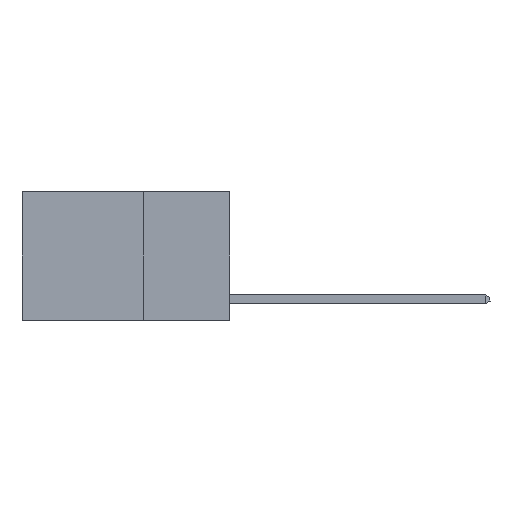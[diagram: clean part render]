
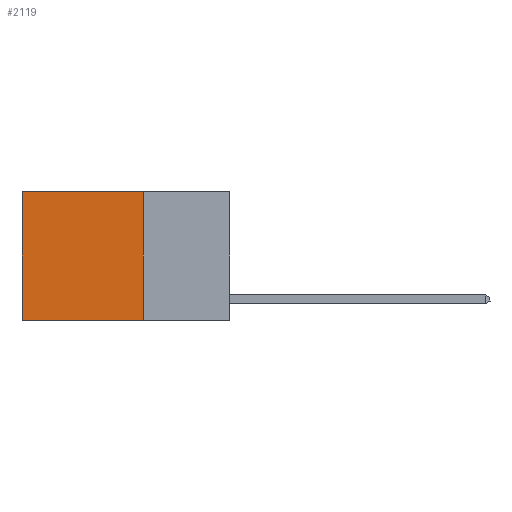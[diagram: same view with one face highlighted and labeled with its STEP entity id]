
A CAD part, left-side view. The second image highlights one B-rep face of the part: STEP entity #2119.
In plain terms, the highlighted planar face has unit normal (-1, 0, 0).
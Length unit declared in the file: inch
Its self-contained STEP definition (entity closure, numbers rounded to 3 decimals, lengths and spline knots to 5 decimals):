
#32 = EDGE_CURVE ( 'NONE', #3670, #4862, #2466, .T. ) ;
#75 = LINE ( 'NONE', #8526, #9297 ) ;
#230 = CARTESIAN_POINT ( 'NONE',  ( 0.2625, 0.25, 0. ) ) ;
#380 = ORIENTED_EDGE ( 'NONE', *, *, #10421, .T. ) ;
#608 = CARTESIAN_POINT ( 'NONE',  ( 0.2625, 0.25, 0. ) ) ;
#822 = CARTESIAN_POINT ( 'NONE',  ( 0.2625, 0.6, -0.37 ) ) ;
#2119 = ADVANCED_FACE ( 'NONE', ( #2214 ), #14959, .F. ) ;
#2214 = FACE_OUTER_BOUND ( 'NONE', #12227, .T. ) ;
#2344 = VERTEX_POINT ( 'NONE', #12533 ) ;
#2466 = LINE ( 'NONE', #230, #11233 ) ;
#3179 = ORIENTED_EDGE ( 'NONE', *, *, #32, .F. ) ;
#3670 = VERTEX_POINT ( 'NONE', #608 ) ;
#4862 = VERTEX_POINT ( 'NONE', #7454 ) ;
#5857 = ORIENTED_EDGE ( 'NONE', *, *, #8252, .F. ) ;
#5997 = DIRECTION ( 'NONE',  ( 0., 0., -1. ) ) ;
#7454 = CARTESIAN_POINT ( 'NONE',  ( 0.2625, 0.25, -0.37 ) ) ;
#8252 = EDGE_CURVE ( 'NONE', #4862, #12870, #8714, .T. ) ;
#8337 = VECTOR ( 'NONE', #13116, 39.37008 ) ;
#8526 = CARTESIAN_POINT ( 'NONE',  ( 0.2625, 0.25, 0. ) ) ;
#8714 = LINE ( 'NONE', #15372, #8337 ) ;
#9297 = VECTOR ( 'NONE', #14390, 39.37008 ) ;
#9470 = LINE ( 'NONE', #14823, #14952 ) ;
#10093 = EDGE_CURVE ( 'NONE', #3670, #2344, #75, .T. ) ;
#10197 = AXIS2_PLACEMENT_3D ( 'NONE', #15402, #14875, #14843 ) ;
#10421 = EDGE_CURVE ( 'NONE', #2344, #12870, #9470, .T. ) ;
#11233 = VECTOR ( 'NONE', #5997, 39.37008 ) ;
#11511 = ORIENTED_EDGE ( 'NONE', *, *, #10093, .T. ) ;
#12227 = EDGE_LOOP ( 'NONE', ( #380, #5857, #3179, #11511 ) ) ;
#12533 = CARTESIAN_POINT ( 'NONE',  ( 0.2625, 0.6, 0. ) ) ;
#12595 = DIRECTION ( 'NONE',  ( 0., 0., -1. ) ) ;
#12870 = VERTEX_POINT ( 'NONE', #822 ) ;
#13116 = DIRECTION ( 'NONE',  ( 0., 1., 0. ) ) ;
#14390 = DIRECTION ( 'NONE',  ( 0., 1., 0. ) ) ;
#14823 = CARTESIAN_POINT ( 'NONE',  ( 0.2625, 0.6, 0. ) ) ;
#14843 = DIRECTION ( 'NONE',  ( 0., 0., -1. ) ) ;
#14875 = DIRECTION ( 'NONE',  ( 1., 0., 0. ) ) ;
#14952 = VECTOR ( 'NONE', #12595, 39.37008 ) ;
#14959 = PLANE ( 'NONE',  #10197 ) ;
#15372 = CARTESIAN_POINT ( 'NONE',  ( 0.2625, 0.25, -0.37 ) ) ;
#15402 = CARTESIAN_POINT ( 'NONE',  ( 0.2625, 0.25, 0. ) ) ;
